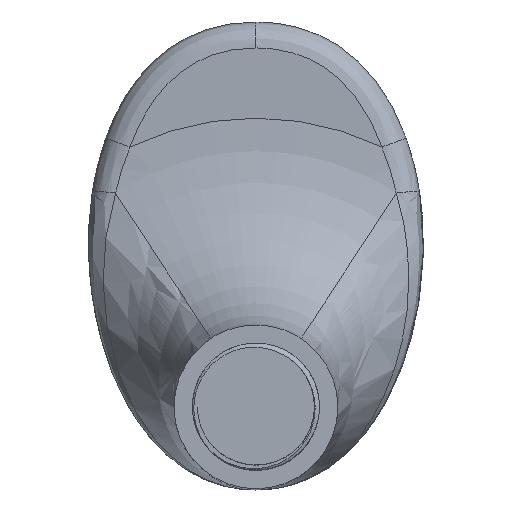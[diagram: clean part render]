
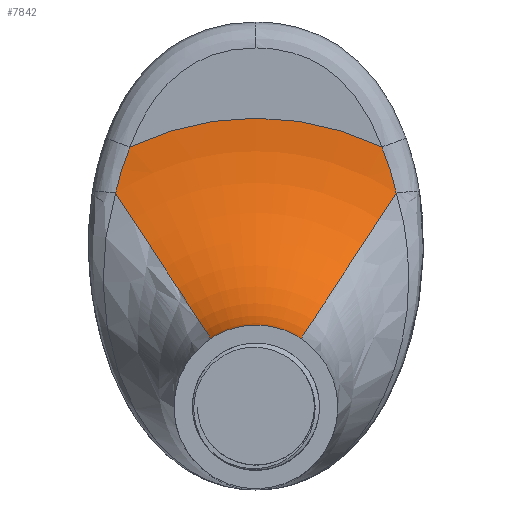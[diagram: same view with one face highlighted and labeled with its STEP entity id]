
A CAD part, top view. The second image highlights one B-rep face of the part: STEP entity #7842.
In plain terms, the highlighted toroidal (fillet/blend) face has major radius 70.8 mm and minor radius 50.8 mm.
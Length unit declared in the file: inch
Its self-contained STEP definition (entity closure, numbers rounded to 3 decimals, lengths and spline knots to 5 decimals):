
#90 = VERTEX_POINT ( 'NONE', #16547 ) ;
#473 = CARTESIAN_POINT ( 'NONE',  ( 1.31296, 1.52217, -8.27892 ) ) ;
#623 = CARTESIAN_POINT ( 'NONE',  ( -1.31296, 1.52217, -8.27892 ) ) ;
#974 = VERTEX_POINT ( 'NONE', #7466 ) ;
#1862 = DIRECTION ( 'NONE',  ( 1., 0., 0. ) ) ;
#2399 = CARTESIAN_POINT ( 'NONE',  ( 1.24063, 1.74313, -8.2893 ) ) ;
#2543 = CARTESIAN_POINT ( 'NONE',  ( -1.34905, 1.37154, -8.26375 ) ) ;
#2559 = DIRECTION ( 'NONE',  ( 0.546, 0.837, 0. ) ) ;
#4042 = EDGE_CURVE ( 'NONE', #12545, #18396, #18114, .T. ) ;
#4328 = CARTESIAN_POINT ( 'NONE',  ( 1.34905, 1.37154, -8.26375 ) ) ;
#4439 = EDGE_CURVE ( 'NONE', #20063, #974, #15594, .T. ) ;
#4738 = CIRCLE ( 'NONE', #21341, 0.7874 ) ;
#5108 = ORIENTED_EDGE ( 'NONE', *, *, #4042, .T. ) ;
#5552 = DIRECTION ( 'NONE',  ( 1., 0., 0. ) ) ;
#6760 = CARTESIAN_POINT ( 'NONE',  ( 0.43028, -0.03656, -6.2893 ) ) ;
#6795 = FACE_OUTER_BOUND ( 'NONE', #20371, .T. ) ;
#7466 = CARTESIAN_POINT ( 'NONE',  ( -1.34905, 1.37154, -8.26375 ) ) ;
#7842 = ADVANCED_FACE ( 'NONE', ( #6795 ), #13429, .F. ) ;
#8290 = CARTESIAN_POINT ( 'NONE',  ( -1.24063, 1.74313, -8.2893 ) ) ;
#9346 = ORIENTED_EDGE ( 'NONE', *, *, #4439, .F. ) ;
#10076 = CARTESIAN_POINT ( 'NONE',  ( 1.34905, 1.37154, -8.26375 ) ) ;
#10908 = EDGE_CURVE ( 'NONE', #21283, #90, #24891, .T. ) ;
#11102 = DIRECTION ( 'NONE',  ( 0., 0., -1. ) ) ;
#11720 = EDGE_CURVE ( 'NONE', #12545, #20063, #4738, .T. ) ;
#12150 = CARTESIAN_POINT ( 'NONE',  ( -1.26702, 1.67011, -8.28731 ) ) ;
#12545 = VERTEX_POINT ( 'NONE', #6760 ) ;
#12770 = B_SPLINE_CURVE_WITH_KNOTS ( 'NONE', 3,
 ( #10076, #21515, #473, #13950, #2399, #15897 ),
 .UNSPECIFIED., .F., .F.,
 ( 4, 2, 4 ),
 ( 0., 0.00591, 0.01182 ),
 .UNSPECIFIED. ) ;
#13144 = CARTESIAN_POINT ( 'NONE',  ( 0., -0.696, -6.2893 ) ) ;
#13389 = DIRECTION ( 'NONE',  ( 0., 0., 1. ) ) ;
#13429 = TOROIDAL_SURFACE ( 'NONE', #22685, 2.7874, 2. ) ;
#13950 = CARTESIAN_POINT ( 'NONE',  ( 1.26702, 1.67011, -8.28731 ) ) ;
#14036 = ORIENTED_EDGE ( 'NONE', *, *, #10908, .F. ) ;
#14091 = CARTESIAN_POINT ( 'NONE',  ( -1.33251, 1.44726, -8.27253 ) ) ;
#14109 = CARTESIAN_POINT ( 'NONE',  ( 1.52319, 1.63842, -6.2893 ) ) ;
#15169 = DIRECTION ( 'NONE',  ( 0., 0., 1. ) ) ;
#15594 = CIRCLE ( 'NONE', #24964, 2. ) ;
#15897 = CARTESIAN_POINT ( 'NONE',  ( 1.21017, 1.815, -8.2893 ) ) ;
#16547 = CARTESIAN_POINT ( 'NONE',  ( 1.21017, 1.815, -8.2893 ) ) ;
#18114 = CIRCLE ( 'NONE', #21451, 2. ) ;
#18215 = EDGE_CURVE ( 'NONE', #18396, #90, #12770, .T. ) ;
#18233 = CARTESIAN_POINT ( 'NONE',  ( -1.21017, 1.815, -8.2893 ) ) ;
#18396 = VERTEX_POINT ( 'NONE', #4328 ) ;
#18855 = ORIENTED_EDGE ( 'NONE', *, *, #11720, .F. ) ;
#19017 = DIRECTION ( 'NONE',  ( -0.546, 0.837, 0. ) ) ;
#19037 = DIRECTION ( 'NONE',  ( 0.837, 0.546, 0. ) ) ;
#19043 = CARTESIAN_POINT ( 'NONE',  ( -1.52319, 1.63842, -6.2893 ) ) ;
#19857 = ORIENTED_EDGE ( 'NONE', *, *, #21849, .T. ) ;
#19869 = CARTESIAN_POINT ( 'NONE',  ( -0.43028, -0.03656, -6.2893 ) ) ;
#19945 = AXIS2_PLACEMENT_3D ( 'NONE', #22624, #11102, #24553 ) ;
#20063 = VERTEX_POINT ( 'NONE', #19869 ) ;
#20351 = ORIENTED_EDGE ( 'NONE', *, *, #18215, .T. ) ;
#20371 = EDGE_LOOP ( 'NONE', ( #14036, #19857, #9346, #18855, #5108, #20351 ) ) ;
#21283 = VERTEX_POINT ( 'NONE', #18233 ) ;
#21341 = AXIS2_PLACEMENT_3D ( 'NONE', #24892, #13389, #1862 ) ;
#21451 = AXIS2_PLACEMENT_3D ( 'NONE', #14109, #21993, #2559 ) ;
#21515 = CARTESIAN_POINT ( 'NONE',  ( 1.33251, 1.44726, -8.27253 ) ) ;
#21740 = CARTESIAN_POINT ( 'NONE',  ( -1.21017, 1.815, -8.2893 ) ) ;
#21849 = EDGE_CURVE ( 'NONE', #21283, #974, #24137, .T. ) ;
#21993 = DIRECTION ( 'NONE',  ( 0.837, -0.546, 0. ) ) ;
#22624 = CARTESIAN_POINT ( 'NONE',  ( 0., -0.696, -8.2893 ) ) ;
#22685 = AXIS2_PLACEMENT_3D ( 'NONE', #13144, #15169, #5552 ) ;
#24137 = B_SPLINE_CURVE_WITH_KNOTS ( 'NONE', 3,
 ( #21740, #8290, #12150, #623, #14091, #2543 ),
 .UNSPECIFIED., .F., .F.,
 ( 4, 2, 4 ),
 ( 0., 0.00591, 0.01182 ),
 .UNSPECIFIED. ) ;
#24553 = DIRECTION ( 'NONE',  ( 1., 0., 0. ) ) ;
#24891 = CIRCLE ( 'NONE', #19945, 2.7874 ) ;
#24892 = CARTESIAN_POINT ( 'NONE',  ( 0., -0.696, -6.2893 ) ) ;
#24964 = AXIS2_PLACEMENT_3D ( 'NONE', #19043, #19037, #19017 ) ;
